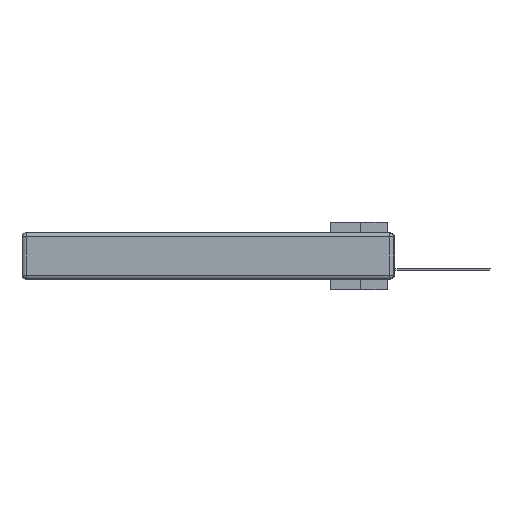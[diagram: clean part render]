
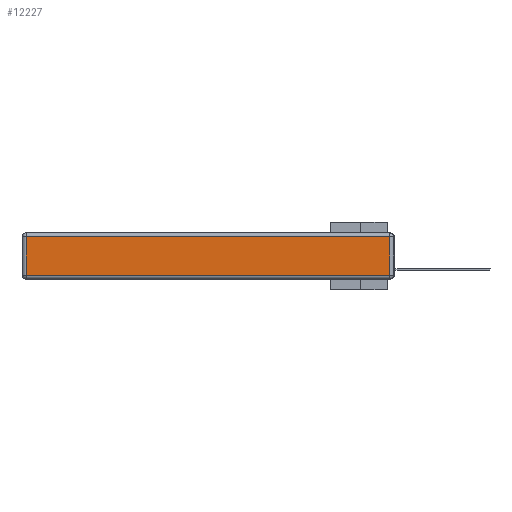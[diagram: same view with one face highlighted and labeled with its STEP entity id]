
A CAD part, left-side view. The second image highlights one B-rep face of the part: STEP entity #12227.
In plain terms, the highlighted planar face has unit normal (-1, 0, 0).
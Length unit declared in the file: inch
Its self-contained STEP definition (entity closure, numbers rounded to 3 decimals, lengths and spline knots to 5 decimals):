
#970 = VECTOR ( 'NONE', #37890, 39.37008 ) ;
#1774 = CARTESIAN_POINT ( 'NONE',  ( 0., 0.03, -0.343 ) ) ;
#1871 = CARTESIAN_POINT ( 'NONE',  ( 0., 0.03, -0.313 ) ) ;
#3989 = ORIENTED_EDGE ( 'NONE', *, *, #18083, .T. ) ;
#4543 = VERTEX_POINT ( 'NONE', #12363 ) ;
#7794 = DIRECTION ( 'NONE',  ( 0., 0., 1. ) ) ;
#8184 = PLANE ( 'NONE',  #34180 ) ;
#9049 = LINE ( 'NONE', #1774, #970 ) ;
#9122 = LINE ( 'NONE', #32809, #23438 ) ;
#10195 = LINE ( 'NONE', #38016, #31622 ) ;
#11199 = ORIENTED_EDGE ( 'NONE', *, *, #33517, .T. ) ;
#12227 = ADVANCED_FACE ( 'NONE', ( #37622 ), #8184, .T. ) ;
#12363 = CARTESIAN_POINT ( 'NONE',  ( 0., 2.72, -0.03 ) ) ;
#12660 = DIRECTION ( 'NONE',  ( 0., 0., -1. ) ) ;
#16348 = VECTOR ( 'NONE', #12660, 39.37008 ) ;
#17065 = ORIENTED_EDGE ( 'NONE', *, *, #23217, .T. ) ;
#18083 = EDGE_CURVE ( 'NONE', #24086, #4543, #10195, .T. ) ;
#18671 = VERTEX_POINT ( 'NONE', #1871 ) ;
#20099 = EDGE_CURVE ( 'NONE', #38277, #18671, #9122, .T. ) ;
#21963 = CARTESIAN_POINT ( 'NONE',  ( 0., 2.72, -0.313 ) ) ;
#23217 = EDGE_CURVE ( 'NONE', #4543, #38277, #35449, .T. ) ;
#23438 = VECTOR ( 'NONE', #39068, 39.37008 ) ;
#24086 = VERTEX_POINT ( 'NONE', #37215 ) ;
#28691 = DIRECTION ( 'NONE',  ( 0., 1., 0. ) ) ;
#29228 = CARTESIAN_POINT ( 'NONE',  ( 0., 0., -0.343 ) ) ;
#30879 = CARTESIAN_POINT ( 'NONE',  ( 0., 2.72, -0.343 ) ) ;
#31622 = VECTOR ( 'NONE', #28691, 39.37008 ) ;
#32809 = CARTESIAN_POINT ( 'NONE',  ( 0., 0., -0.313 ) ) ;
#33517 = EDGE_CURVE ( 'NONE', #18671, #24086, #9049, .T. ) ;
#34180 = AXIS2_PLACEMENT_3D ( 'NONE', #29228, #38678, #7794 ) ;
#35449 = LINE ( 'NONE', #30879, #16348 ) ;
#37215 = CARTESIAN_POINT ( 'NONE',  ( 0., 0.03, -0.03 ) ) ;
#37622 = FACE_OUTER_BOUND ( 'NONE', #38952, .T. ) ;
#37788 = ORIENTED_EDGE ( 'NONE', *, *, #20099, .T. ) ;
#37890 = DIRECTION ( 'NONE',  ( 0., 0., 1. ) ) ;
#38016 = CARTESIAN_POINT ( 'NONE',  ( 0., 2.75, -0.03 ) ) ;
#38277 = VERTEX_POINT ( 'NONE', #21963 ) ;
#38678 = DIRECTION ( 'NONE',  ( -1., 0., 0. ) ) ;
#38952 = EDGE_LOOP ( 'NONE', ( #37788, #11199, #3989, #17065 ) ) ;
#39068 = DIRECTION ( 'NONE',  ( 0., -1., 0. ) ) ;
